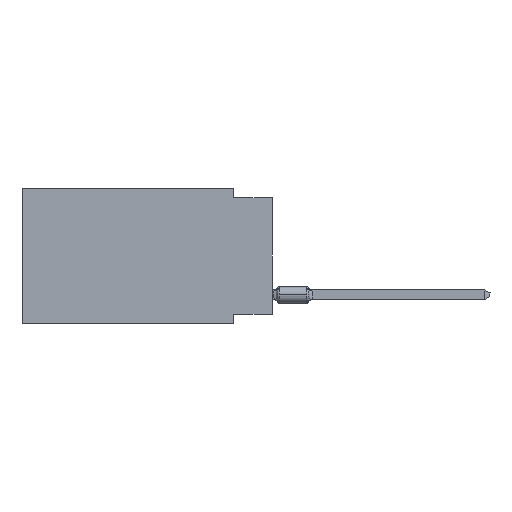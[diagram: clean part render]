
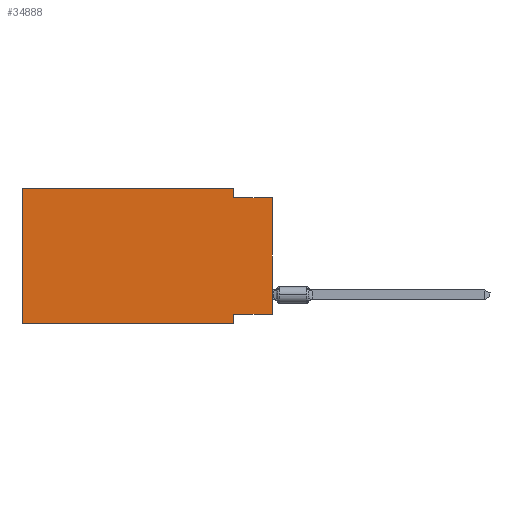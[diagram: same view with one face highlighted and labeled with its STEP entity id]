
A CAD part, left-side view. The second image highlights one B-rep face of the part: STEP entity #34888.
In plain terms, the highlighted planar face has unit normal (-1, 0, 0).
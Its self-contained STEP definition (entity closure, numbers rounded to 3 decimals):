
#750 = EDGE_CURVE ( 'NONE', #54708, #25285, #19832, .T. ) ;
#2451 = EDGE_LOOP ( 'NONE', ( #3382, #4437, #7956, #38335, #40005, #57546, #35305, #13854 ) ) ;
#3382 = ORIENTED_EDGE ( 'NONE', *, *, #77816, .T. ) ;
#4064 = CARTESIAN_POINT ( 'NONE',  ( 0., 16.383, 0. ) ) ;
#4437 = ORIENTED_EDGE ( 'NONE', *, *, #45112, .F. ) ;
#5053 = VECTOR ( 'NONE', #7243, 1000. ) ;
#7243 = DIRECTION ( 'NONE',  ( 0., 1., 0. ) ) ;
#7956 = ORIENTED_EDGE ( 'NONE', *, *, #63285, .F. ) ;
#9399 = DIRECTION ( 'NONE',  ( 0., 0., 1. ) ) ;
#9555 = LINE ( 'NONE', #23390, #43811 ) ;
#11073 = EDGE_CURVE ( 'NONE', #24971, #38879, #42530, .T. ) ;
#13148 = DIRECTION ( 'NONE',  ( 0., 0., -1. ) ) ;
#13854 = ORIENTED_EDGE ( 'NONE', *, *, #750, .F. ) ;
#14721 = CARTESIAN_POINT ( 'NONE',  ( 0., 2.54, 0. ) ) ;
#14759 = DIRECTION ( 'NONE',  ( 1., 0., 0. ) ) ;
#15167 = FACE_OUTER_BOUND ( 'NONE', #2451, .T. ) ;
#18059 = CARTESIAN_POINT ( 'NONE',  ( 0., 2.54, -8.89 ) ) ;
#19832 = LINE ( 'NONE', #32428, #5053 ) ;
#19989 = LINE ( 'NONE', #31764, #82356 ) ;
#20414 = CARTESIAN_POINT ( 'NONE',  ( 0., 2.54, -8.89 ) ) ;
#21459 = DIRECTION ( 'NONE',  ( 0., 0., -1. ) ) ;
#23390 = CARTESIAN_POINT ( 'NONE',  ( 0., 0., 0. ) ) ;
#24971 = VERTEX_POINT ( 'NONE', #65001 ) ;
#25285 = VERTEX_POINT ( 'NONE', #33375 ) ;
#26154 = CARTESIAN_POINT ( 'NONE',  ( 0., 2.54, 0. ) ) ;
#26207 = AXIS2_PLACEMENT_3D ( 'NONE', #58401, #14759, #21459 ) ;
#28430 = LINE ( 'NONE', #60316, #39731 ) ;
#29691 = DIRECTION ( 'NONE',  ( 0., 0., 1. ) ) ;
#30090 = VECTOR ( 'NONE', #9399, 1000. ) ;
#31764 = CARTESIAN_POINT ( 'NONE',  ( 0., 16.383, -8.89 ) ) ;
#31769 = DIRECTION ( 'NONE',  ( 0., 0., -1. ) ) ;
#32428 = CARTESIAN_POINT ( 'NONE',  ( 0., 0., -8.255 ) ) ;
#33375 = CARTESIAN_POINT ( 'NONE',  ( 0., 2.54, -8.255 ) ) ;
#33837 = EDGE_CURVE ( 'NONE', #24971, #79144, #19989, .T. ) ;
#34888 = ADVANCED_FACE ( 'NONE', ( #15167 ), #79359, .F. ) ;
#35120 = LINE ( 'NONE', #4064, #74434 ) ;
#35122 = VECTOR ( 'NONE', #13148, 1000. ) ;
#35305 = ORIENTED_EDGE ( 'NONE', *, *, #47752, .F. ) ;
#38335 = ORIENTED_EDGE ( 'NONE', *, *, #55039, .F. ) ;
#38461 = DIRECTION ( 'NONE',  ( 0., -1., 0. ) ) ;
#38665 = CARTESIAN_POINT ( 'NONE',  ( 0., 16.383, 0. ) ) ;
#38879 = VERTEX_POINT ( 'NONE', #38665 ) ;
#39731 = VECTOR ( 'NONE', #65367, 1000. ) ;
#40005 = ORIENTED_EDGE ( 'NONE', *, *, #11073, .F. ) ;
#41757 = VERTEX_POINT ( 'NONE', #55778 ) ;
#42116 = CARTESIAN_POINT ( 'NONE',  ( 0., 16.383, 0. ) ) ;
#42530 = LINE ( 'NONE', #42116, #30090 ) ;
#43759 = VERTEX_POINT ( 'NONE', #66933 ) ;
#43811 = VECTOR ( 'NONE', #29691, 1000. ) ;
#45112 = EDGE_CURVE ( 'NONE', #41757, #43759, #28430, .T. ) ;
#47752 = EDGE_CURVE ( 'NONE', #25285, #79144, #69959, .T. ) ;
#54708 = VERTEX_POINT ( 'NONE', #67957 ) ;
#55039 = EDGE_CURVE ( 'NONE', #38879, #63843, #35120, .T. ) ;
#55778 = CARTESIAN_POINT ( 'NONE',  ( 0., 2.54, -0.635 ) ) ;
#57546 = ORIENTED_EDGE ( 'NONE', *, *, #33837, .T. ) ;
#58401 = CARTESIAN_POINT ( 'NONE',  ( 0., 16.383, 0. ) ) ;
#58455 = LINE ( 'NONE', #26154, #35122 ) ;
#60316 = CARTESIAN_POINT ( 'NONE',  ( 0., 0., -0.635 ) ) ;
#63285 = EDGE_CURVE ( 'NONE', #63843, #41757, #58455, .T. ) ;
#63843 = VERTEX_POINT ( 'NONE', #14721 ) ;
#65001 = CARTESIAN_POINT ( 'NONE',  ( 0., 16.383, -8.89 ) ) ;
#65367 = DIRECTION ( 'NONE',  ( 0., -1., 0. ) ) ;
#66933 = CARTESIAN_POINT ( 'NONE',  ( 0., 0., -0.635 ) ) ;
#67957 = CARTESIAN_POINT ( 'NONE',  ( 0., 0., -8.255 ) ) ;
#69959 = LINE ( 'NONE', #20414, #70824 ) ;
#70824 = VECTOR ( 'NONE', #31769, 1000. ) ;
#74434 = VECTOR ( 'NONE', #80858, 1000. ) ;
#77816 = EDGE_CURVE ( 'NONE', #54708, #43759, #9555, .T. ) ;
#79144 = VERTEX_POINT ( 'NONE', #18059 ) ;
#79359 = PLANE ( 'NONE',  #26207 ) ;
#80858 = DIRECTION ( 'NONE',  ( 0., -1., 0. ) ) ;
#82356 = VECTOR ( 'NONE', #38461, 1000. ) ;
